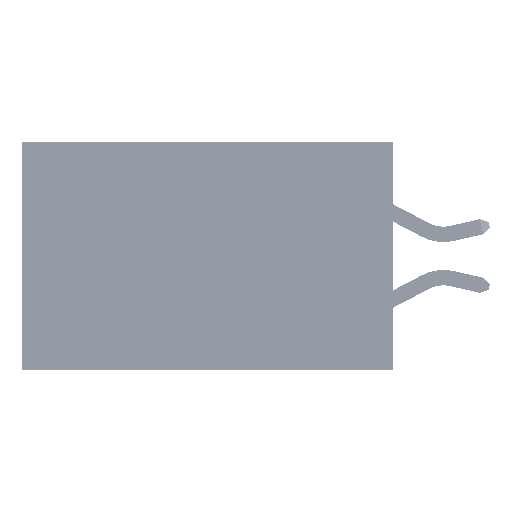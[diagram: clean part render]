
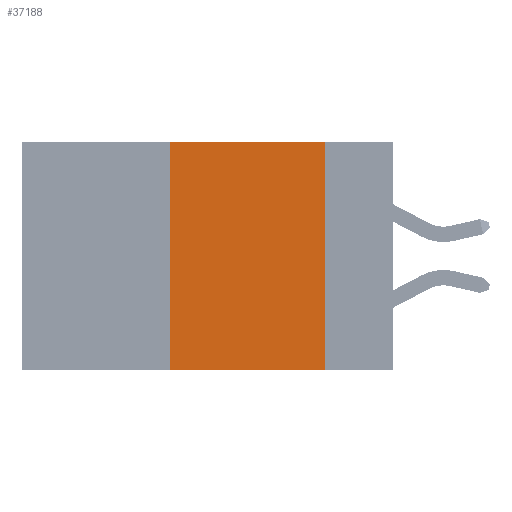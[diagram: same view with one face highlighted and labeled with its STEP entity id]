
A CAD part, left-side view. The second image highlights one B-rep face of the part: STEP entity #37188.
In plain terms, the highlighted planar face has unit normal (-1, 0, 0).
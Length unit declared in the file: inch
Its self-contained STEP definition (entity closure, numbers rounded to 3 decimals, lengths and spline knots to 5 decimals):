
#67 = DIRECTION ( 'NONE',  ( 0., -1., 0. ) ) ;
#507 = CARTESIAN_POINT ( 'NONE',  ( 0., 0.6, 0. ) ) ;
#3455 = LINE ( 'NONE', #3972, #9126 ) ;
#3589 = EDGE_CURVE ( 'NONE', #50257, #28299, #3455, .T. ) ;
#3670 = EDGE_CURVE ( 'NONE', #39234, #50257, #40850, .T. ) ;
#3972 = CARTESIAN_POINT ( 'NONE',  ( 0., 0.6, 0. ) ) ;
#3990 = CARTESIAN_POINT ( 'NONE',  ( 0., 0.11, -0.37 ) ) ;
#4142 = PLANE ( 'NONE',  #47459 ) ;
#5520 = CARTESIAN_POINT ( 'NONE',  ( 0., 0.36, 0. ) ) ;
#8920 = ORIENTED_EDGE ( 'NONE', *, *, #3589, .F. ) ;
#9126 = VECTOR ( 'NONE', #67, 39.37008 ) ;
#12426 = LINE ( 'NONE', #20499, #32868 ) ;
#12795 = EDGE_CURVE ( 'NONE', #28299, #48094, #29594, .T. ) ;
#16197 = DIRECTION ( 'NONE',  ( 0., 0., 1. ) ) ;
#18134 = CARTESIAN_POINT ( 'NONE',  ( 0., 0.11, 0. ) ) ;
#18478 = ORIENTED_EDGE ( 'NONE', *, *, #3670, .F. ) ;
#20499 = CARTESIAN_POINT ( 'NONE',  ( 0., 0.6, -0.37 ) ) ;
#21550 = DIRECTION ( 'NONE',  ( 0., 0., -1. ) ) ;
#22256 = EDGE_LOOP ( 'NONE', ( #29236, #8920, #18478, #46221 ) ) ;
#24871 = DIRECTION ( 'NONE',  ( 0., -1., 0. ) ) ;
#28299 = VERTEX_POINT ( 'NONE', #18134 ) ;
#28811 = CARTESIAN_POINT ( 'NONE',  ( 0., 0.36, -0.37 ) ) ;
#29236 = ORIENTED_EDGE ( 'NONE', *, *, #12795, .F. ) ;
#29594 = LINE ( 'NONE', #34237, #32762 ) ;
#32762 = VECTOR ( 'NONE', #21550, 39.37008 ) ;
#32868 = VECTOR ( 'NONE', #24871, 39.37008 ) ;
#34237 = CARTESIAN_POINT ( 'NONE',  ( 0., 0.11, 0. ) ) ;
#35576 = DIRECTION ( 'NONE',  ( 0., 0., -1. ) ) ;
#36099 = FACE_OUTER_BOUND ( 'NONE', #22256, .T. ) ;
#37188 = ADVANCED_FACE ( 'NONE', ( #36099 ), #4142, .F. ) ;
#38857 = CARTESIAN_POINT ( 'NONE',  ( 0., 0.36, 0. ) ) ;
#39234 = VERTEX_POINT ( 'NONE', #28811 ) ;
#39733 = DIRECTION ( 'NONE',  ( 1., 0., 0. ) ) ;
#40850 = LINE ( 'NONE', #5520, #41541 ) ;
#41541 = VECTOR ( 'NONE', #16197, 39.37008 ) ;
#46077 = EDGE_CURVE ( 'NONE', #39234, #48094, #12426, .T. ) ;
#46221 = ORIENTED_EDGE ( 'NONE', *, *, #46077, .T. ) ;
#47459 = AXIS2_PLACEMENT_3D ( 'NONE', #507, #39733, #35576 ) ;
#48094 = VERTEX_POINT ( 'NONE', #3990 ) ;
#50257 = VERTEX_POINT ( 'NONE', #38857 ) ;
